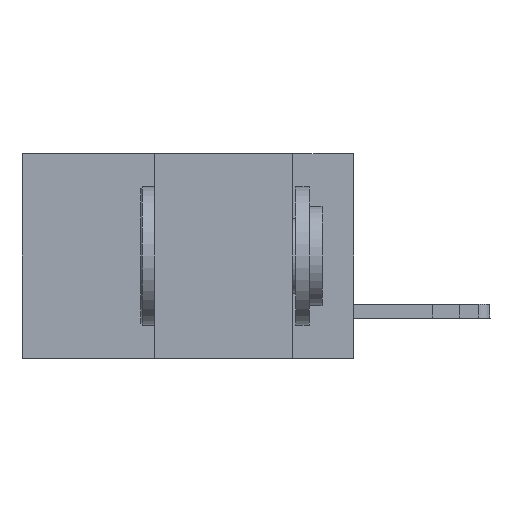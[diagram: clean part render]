
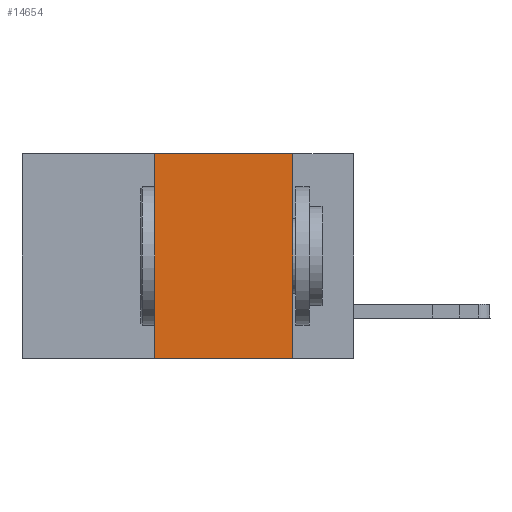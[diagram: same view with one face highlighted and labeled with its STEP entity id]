
A CAD part, left-side view. The second image highlights one B-rep face of the part: STEP entity #14654.
In plain terms, the highlighted planar face has unit normal (-1, 0, 0).
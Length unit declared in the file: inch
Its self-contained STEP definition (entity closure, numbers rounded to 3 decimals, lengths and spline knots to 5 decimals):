
#23 = VERTEX_POINT ( 'NONE', #15332 ) ;
#716 = CARTESIAN_POINT ( 'NONE',  ( 0., 0.6, -0.37 ) ) ;
#1213 = ORIENTED_EDGE ( 'NONE', *, *, #4473, .F. ) ;
#1383 = CARTESIAN_POINT ( 'NONE',  ( 0., 0.6, 0. ) ) ;
#1595 = DIRECTION ( 'NONE',  ( 0., -1., 0. ) ) ;
#2244 = DIRECTION ( 'NONE',  ( 0., 0., -1. ) ) ;
#2508 = CARTESIAN_POINT ( 'NONE',  ( 0., 0.36, -0.37 ) ) ;
#4473 = EDGE_CURVE ( 'NONE', #7716, #23, #20317, .T. ) ;
#6831 = VECTOR ( 'NONE', #9770, 39.37008 ) ;
#7088 = EDGE_LOOP ( 'NONE', ( #12923, #1213, #17395, #19928 ) ) ;
#7519 = VECTOR ( 'NONE', #22101, 39.37008 ) ;
#7716 = VERTEX_POINT ( 'NONE', #14632 ) ;
#9754 = EDGE_CURVE ( 'NONE', #23, #11054, #18834, .T. ) ;
#9770 = DIRECTION ( 'NONE',  ( 0., -1., 0. ) ) ;
#11054 = VERTEX_POINT ( 'NONE', #21507 ) ;
#12426 = FACE_OUTER_BOUND ( 'NONE', #7088, .T. ) ;
#12534 = PLANE ( 'NONE',  #14891 ) ;
#12923 = ORIENTED_EDGE ( 'NONE', *, *, #9754, .F. ) ;
#13100 = LINE ( 'NONE', #15141, #7519 ) ;
#13537 = VERTEX_POINT ( 'NONE', #2508 ) ;
#14103 = DIRECTION ( 'NONE',  ( 1., 0., 0. ) ) ;
#14632 = CARTESIAN_POINT ( 'NONE',  ( 0., 0.36, 0. ) ) ;
#14654 = ADVANCED_FACE ( 'NONE', ( #12426 ), #12534, .F. ) ;
#14891 = AXIS2_PLACEMENT_3D ( 'NONE', #19607, #14103, #2244 ) ;
#14937 = DIRECTION ( 'NONE',  ( 0., 0., -1. ) ) ;
#14950 = LINE ( 'NONE', #716, #6831 ) ;
#15141 = CARTESIAN_POINT ( 'NONE',  ( 0., 0.36, 0. ) ) ;
#15332 = CARTESIAN_POINT ( 'NONE',  ( 0., 0.11, 0. ) ) ;
#16154 = EDGE_CURVE ( 'NONE', #13537, #7716, #13100, .T. ) ;
#16791 = CARTESIAN_POINT ( 'NONE',  ( 0., 0.11, 0. ) ) ;
#17395 = ORIENTED_EDGE ( 'NONE', *, *, #16154, .F. ) ;
#18834 = LINE ( 'NONE', #16791, #19329 ) ;
#19329 = VECTOR ( 'NONE', #14937, 39.37008 ) ;
#19607 = CARTESIAN_POINT ( 'NONE',  ( 0., 0.6, 0. ) ) ;
#19858 = VECTOR ( 'NONE', #1595, 39.37008 ) ;
#19928 = ORIENTED_EDGE ( 'NONE', *, *, #21902, .T. ) ;
#20317 = LINE ( 'NONE', #1383, #19858 ) ;
#21507 = CARTESIAN_POINT ( 'NONE',  ( 0., 0.11, -0.37 ) ) ;
#21902 = EDGE_CURVE ( 'NONE', #13537, #11054, #14950, .T. ) ;
#22101 = DIRECTION ( 'NONE',  ( 0., 0., 1. ) ) ;
